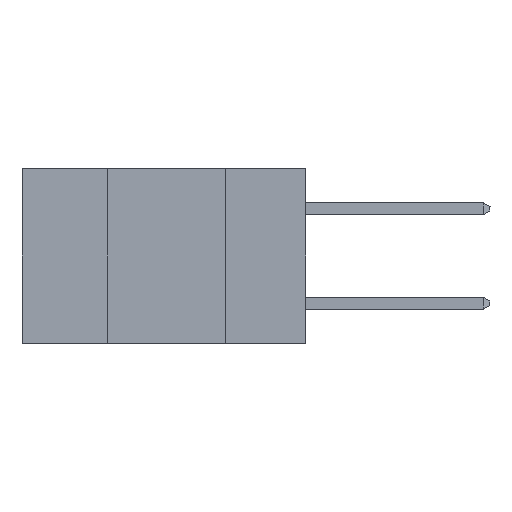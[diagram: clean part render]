
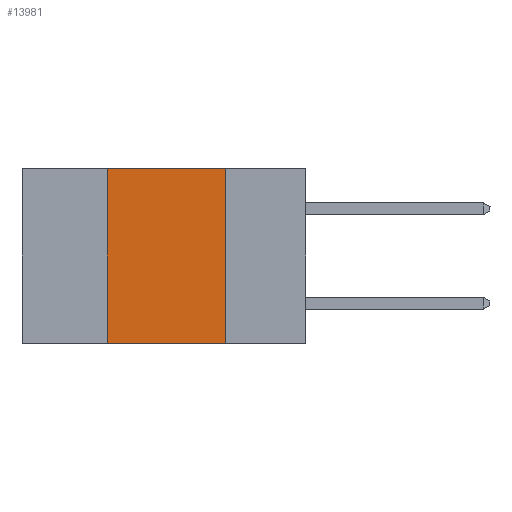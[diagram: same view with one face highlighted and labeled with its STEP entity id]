
A CAD part, left-side view. The second image highlights one B-rep face of the part: STEP entity #13981.
In plain terms, the highlighted planar face has unit normal (-1, 0, 0).
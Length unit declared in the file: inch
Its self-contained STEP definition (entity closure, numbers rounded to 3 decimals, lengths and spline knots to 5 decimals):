
#152 = LINE ( 'NONE', #5669, #10799 ) ;
#799 = VECTOR ( 'NONE', #23114, 39.37008 ) ;
#2369 = LINE ( 'NONE', #5393, #18625 ) ;
#2389 = ORIENTED_EDGE ( 'NONE', *, *, #27136, .F. ) ;
#2550 = ORIENTED_EDGE ( 'NONE', *, *, #5553, .F. ) ;
#5393 = CARTESIAN_POINT ( 'NONE',  ( 0., 0.6, -0.37 ) ) ;
#5412 = CARTESIAN_POINT ( 'NONE',  ( 0., 0.6, 0. ) ) ;
#5553 = EDGE_CURVE ( 'NONE', #12156, #18423, #15712, .T. ) ;
#5669 = CARTESIAN_POINT ( 'NONE',  ( 0., 0.42, -0.37 ) ) ;
#5781 = EDGE_LOOP ( 'NONE', ( #2550, #2389, #6724, #14357 ) ) ;
#6724 = ORIENTED_EDGE ( 'NONE', *, *, #12669, .F. ) ;
#7394 = PLANE ( 'NONE',  #9086 ) ;
#7458 = LINE ( 'NONE', #11564, #23550 ) ;
#7551 = DIRECTION ( 'NONE',  ( 0., -1., 0. ) ) ;
#9086 = AXIS2_PLACEMENT_3D ( 'NONE', #5412, #22283, #9689 ) ;
#9689 = DIRECTION ( 'NONE',  ( 0., 0., -1. ) ) ;
#10799 = VECTOR ( 'NONE', #22525, 39.37008 ) ;
#11564 = CARTESIAN_POINT ( 'NONE',  ( 0., 0.6, 0. ) ) ;
#11586 = VERTEX_POINT ( 'NONE', #21115 ) ;
#12156 = VERTEX_POINT ( 'NONE', #12323 ) ;
#12323 = CARTESIAN_POINT ( 'NONE',  ( 0., 0.17, 0. ) ) ;
#12669 = EDGE_CURVE ( 'NONE', #11586, #15781, #152, .T. ) ;
#13678 = DIRECTION ( 'NONE',  ( 0., -1., 0. ) ) ;
#13981 = ADVANCED_FACE ( 'NONE', ( #21902 ), #7394, .F. ) ;
#14357 = ORIENTED_EDGE ( 'NONE', *, *, #14554, .T. ) ;
#14554 = EDGE_CURVE ( 'NONE', #11586, #18423, #2369, .T. ) ;
#15712 = LINE ( 'NONE', #18963, #799 ) ;
#15781 = VERTEX_POINT ( 'NONE', #21343 ) ;
#16500 = CARTESIAN_POINT ( 'NONE',  ( 0., 0.17, -0.37 ) ) ;
#18423 = VERTEX_POINT ( 'NONE', #16500 ) ;
#18625 = VECTOR ( 'NONE', #7551, 39.37008 ) ;
#18963 = CARTESIAN_POINT ( 'NONE',  ( 0., 0.17, -0.37 ) ) ;
#21115 = CARTESIAN_POINT ( 'NONE',  ( 0., 0.42, -0.37 ) ) ;
#21343 = CARTESIAN_POINT ( 'NONE',  ( 0., 0.42, 0. ) ) ;
#21902 = FACE_OUTER_BOUND ( 'NONE', #5781, .T. ) ;
#22283 = DIRECTION ( 'NONE',  ( 1., 0., 0. ) ) ;
#22525 = DIRECTION ( 'NONE',  ( 0., 0., 1. ) ) ;
#23114 = DIRECTION ( 'NONE',  ( 0., 0., -1. ) ) ;
#23550 = VECTOR ( 'NONE', #13678, 39.37008 ) ;
#27136 = EDGE_CURVE ( 'NONE', #15781, #12156, #7458, .T. ) ;
